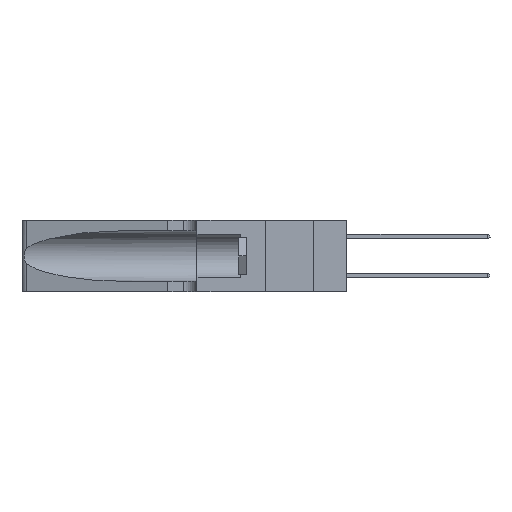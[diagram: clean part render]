
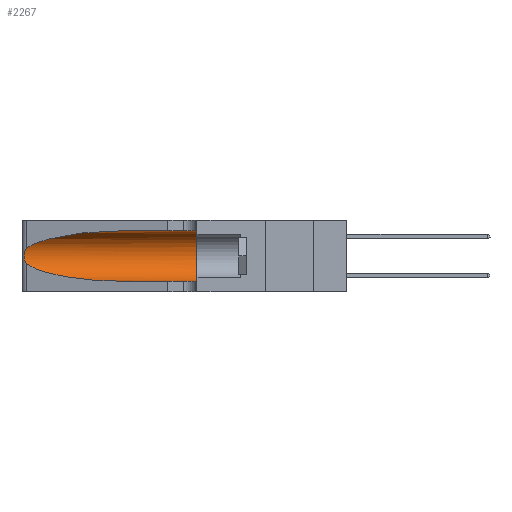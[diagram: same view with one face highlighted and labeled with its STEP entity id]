
A CAD part, left-side view. The second image highlights one B-rep face of the part: STEP entity #2267.
In plain terms, the highlighted cylindrical face has radius 3.308 mm (diameter 6.617 mm), a partial arc.
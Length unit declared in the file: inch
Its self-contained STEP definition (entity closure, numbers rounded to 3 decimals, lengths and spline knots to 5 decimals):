
#313 = VECTOR ( 'NONE', #25745, 39.37008 ) ;
#545 = CARTESIAN_POINT ( 'NONE',  ( 0.25487, 1.22718, 0.22369 ) ) ;
#1054 = CARTESIAN_POINT ( 'NONE',  ( 0.1305, 1.61858, 0.05475 ) ) ;
#1357 = CARTESIAN_POINT ( 'NONE',  ( 0.25555, 1.22993, 0.14849 ) ) ;
#1405 = CARTESIAN_POINT ( 'NONE',  ( 0.1305, 0.72297, 0.31525 ) ) ;
#1653 = ORIENTED_EDGE ( 'NONE', *, *, #10355, .T. ) ;
#2149 = EDGE_LOOP ( 'NONE', ( #19820, #1653, #32853, #24359, #27214, #15914 ) ) ;
#2267 = ADVANCED_FACE ( 'NONE', ( #34830 ), #34333, .F. ) ;
#2789 = CARTESIAN_POINT ( 'NONE',  ( 0.1305, 1.61858, 0.185 ) ) ;
#5047 = AXIS2_PLACEMENT_3D ( 'NONE', #35997, #14328, #39590 ) ;
#5061 = CARTESIAN_POINT ( 'NONE',  ( 0.25487, 1.22718, 0.22369 ) ) ;
#5511 = CIRCLE ( 'NONE', #5047, 0.13025 ) ;
#5879 = EDGE_CURVE ( 'NONE', #6994, #27767, #18788, .T. ) ;
#6875 =( BOUNDED_CURVE ( )  B_SPLINE_CURVE ( 3, ( #9193, #30904, #16479, #41709 ),
 .UNSPECIFIED., .F., .F. ) 
 B_SPLINE_CURVE_WITH_KNOTS ( ( 4, 4 ),
 ( 3.44316, 4.71239 ),
 .UNSPECIFIED. ) 
 CURVE ( )  GEOMETRIC_REPRESENTATION_ITEM ( )  RATIONAL_B_SPLINE_CURVE ( ( 1., 0.87, 0.87, 1. ) ) 
 REPRESENTATION_ITEM ( '' )  );
#6994 = VERTEX_POINT ( 'NONE', #43516 ) ;
#7797 = LINE ( 'NONE', #1054, #35535 ) ;
#8465 = CARTESIAN_POINT ( 'NONE',  ( 0.1305, 0.35, 0.31525 ) ) ;
#8522 = CARTESIAN_POINT ( 'NONE',  ( 0.25787, 1.23484, 0.2124 ) ) ;
#9164 = CARTESIAN_POINT ( 'NONE',  ( 0.25487, 1.22718, 0.22369 ) ) ;
#9193 = CARTESIAN_POINT ( 'NONE',  ( 0.25487, 1.22718, 0.14631 ) ) ;
#10009 = LINE ( 'NONE', #29247, #313 ) ;
#10109 = DIRECTION ( 'NONE',  ( 0., -1., 0. ) ) ;
#10355 = EDGE_CURVE ( 'NONE', #27767, #13916, #40479, .T. ) ;
#11061 = VERTEX_POINT ( 'NONE', #8465 ) ;
#12139 = CARTESIAN_POINT ( 'NONE',  ( 0.26018, 1.23835, 0.19895 ) ) ;
#12214 = VERTEX_POINT ( 'NONE', #40130 ) ;
#13916 = VERTEX_POINT ( 'NONE', #22760 ) ;
#14328 = DIRECTION ( 'NONE',  ( 0., 1., 0. ) ) ;
#15800 = CARTESIAN_POINT ( 'NONE',  ( 0.26075, 1.23896, 0.178 ) ) ;
#15914 = ORIENTED_EDGE ( 'NONE', *, *, #26289, .F. ) ;
#16479 = CARTESIAN_POINT ( 'NONE',  ( 0.18966, 0.96281, 0.05475 ) ) ;
#18788 =( BOUNDED_CURVE ( )  B_SPLINE_CURVE ( 3, ( #1405, #23114, #26765, #5061 ),
 .UNSPECIFIED., .F., .F. ) 
 B_SPLINE_CURVE_WITH_KNOTS ( ( 4, 4 ),
 ( 1.5708, 2.84003 ),
 .UNSPECIFIED. ) 
 CURVE ( )  GEOMETRIC_REPRESENTATION_ITEM ( )  RATIONAL_B_SPLINE_CURVE ( ( 1., 0.87, 0.87, 1. ) ) 
 REPRESENTATION_ITEM ( '' )  );
#19455 = CARTESIAN_POINT ( 'NONE',  ( 0.25856, 1.23593, 0.16098 ) ) ;
#19820 = ORIENTED_EDGE ( 'NONE', *, *, #5879, .T. ) ;
#20763 = EDGE_CURVE ( 'NONE', #12214, #36704, #7797, .T. ) ;
#22760 = CARTESIAN_POINT ( 'NONE',  ( 0.25487, 1.22718, 0.14631 ) ) ;
#23063 = CARTESIAN_POINT ( 'NONE',  ( 0.25639, 1.23186, 0.15144 ) ) ;
#23114 = CARTESIAN_POINT ( 'NONE',  ( 0.18966, 0.96281, 0.31525 ) ) ;
#24263 = EDGE_CURVE ( 'NONE', #13916, #12214, #6875, .T. ) ;
#24359 = ORIENTED_EDGE ( 'NONE', *, *, #20763, .T. ) ;
#25745 = DIRECTION ( 'NONE',  ( 0., -1., 0. ) ) ;
#25919 = AXIS2_PLACEMENT_3D ( 'NONE', #2789, #10109, #31808 ) ;
#26289 = EDGE_CURVE ( 'NONE', #6994, #11061, #10009, .T. ) ;
#26556 = CARTESIAN_POINT ( 'NONE',  ( 0.25555, 1.22994, 0.2215 ) ) ;
#26718 = CARTESIAN_POINT ( 'NONE',  ( 0.25487, 1.22718, 0.14631 ) ) ;
#26765 = CARTESIAN_POINT ( 'NONE',  ( 0.2373, 1.15595, 0.28018 ) ) ;
#27214 = ORIENTED_EDGE ( 'NONE', *, *, #42841, .F. ) ;
#27767 = VERTEX_POINT ( 'NONE', #9164 ) ;
#29132 = CARTESIAN_POINT ( 'NONE',  ( 0.1305, 0.35, 0.05475 ) ) ;
#29247 = CARTESIAN_POINT ( 'NONE',  ( 0.1305, 1.61858, 0.31525 ) ) ;
#30219 = CARTESIAN_POINT ( 'NONE',  ( 0.25639, 1.23184, 0.21858 ) ) ;
#30904 = CARTESIAN_POINT ( 'NONE',  ( 0.2373, 1.15595, 0.08982 ) ) ;
#31808 = DIRECTION ( 'NONE',  ( 0., 0., -1. ) ) ;
#32853 = ORIENTED_EDGE ( 'NONE', *, *, #24263, .T. ) ;
#33693 = DIRECTION ( 'NONE',  ( 0., -1., 0. ) ) ;
#33831 = CARTESIAN_POINT ( 'NONE',  ( 0.25854, 1.2359, 0.20912 ) ) ;
#34333 = CYLINDRICAL_SURFACE ( 'NONE', #25919, 0.13025 ) ;
#34830 = FACE_OUTER_BOUND ( 'NONE', #2149, .T. ) ;
#35535 = VECTOR ( 'NONE', #33693, 39.37008 ) ;
#35997 = CARTESIAN_POINT ( 'NONE',  ( 0.1305, 0.35, 0.185 ) ) ;
#36704 = VERTEX_POINT ( 'NONE', #29132 ) ;
#37469 = CARTESIAN_POINT ( 'NONE',  ( 0.26075, 1.23896, 0.19203 ) ) ;
#39590 = DIRECTION ( 'NONE',  ( 0., 0., 1. ) ) ;
#40130 = CARTESIAN_POINT ( 'NONE',  ( 0.1305, 0.72297, 0.05475 ) ) ;
#40479 = B_SPLINE_CURVE_WITH_KNOTS ( 'NONE', 3,
 ( #545, #26556, #30219, #8522, #33831, #12139, #37469, #15800, #41053, #19455, #44637, #23063, #1357, #26718 ),
 .UNSPECIFIED., .F., .F.,
 ( 4, 2, 2, 2, 2, 2, 4 ),
 ( 0., 0.00027, 0.00053, 0.00107, 0.0016, 0.00187, 0.00214 ),
 .UNSPECIFIED. ) ;
#41053 = CARTESIAN_POINT ( 'NONE',  ( 0.26017, 1.23833, 0.17102 ) ) ;
#41709 = CARTESIAN_POINT ( 'NONE',  ( 0.1305, 0.72297, 0.05475 ) ) ;
#42841 = EDGE_CURVE ( 'NONE', #11061, #36704, #5511, .T. ) ;
#43516 = CARTESIAN_POINT ( 'NONE',  ( 0.1305, 0.72297, 0.31525 ) ) ;
#44637 = CARTESIAN_POINT ( 'NONE',  ( 0.25789, 1.23486, 0.15765 ) ) ;
